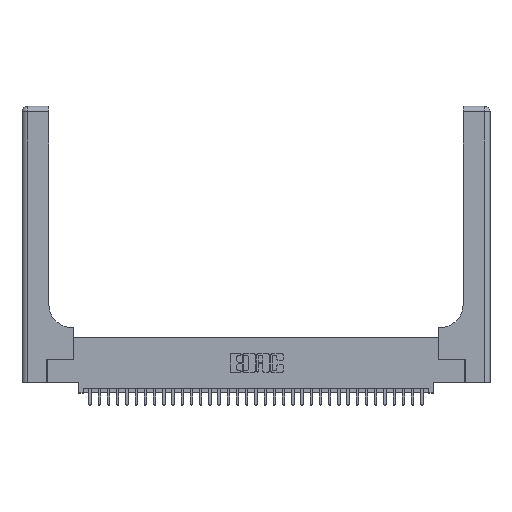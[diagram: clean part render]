
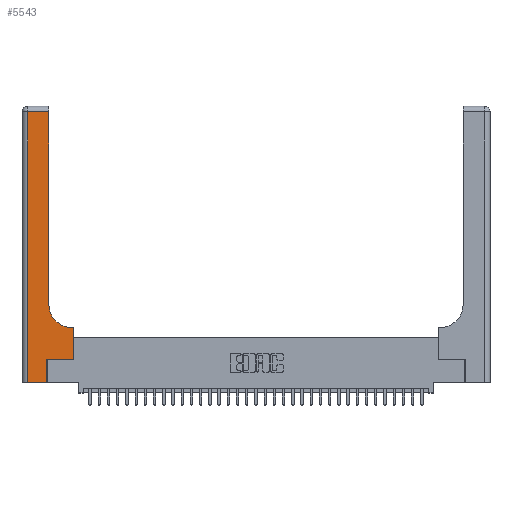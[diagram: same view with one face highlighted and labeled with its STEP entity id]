
A CAD part, top view. The second image highlights one B-rep face of the part: STEP entity #5543.
In plain terms, the highlighted planar face has unit normal (0, 0, 1).
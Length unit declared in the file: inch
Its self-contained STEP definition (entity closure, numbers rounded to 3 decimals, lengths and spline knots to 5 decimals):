
#311 = VECTOR ( 'NONE', #27651, 39.37008 ) ;
#631 = ORIENTED_EDGE ( 'NONE', *, *, #18837, .T. ) ;
#1269 = ORIENTED_EDGE ( 'NONE', *, *, #34056, .T. ) ;
#2179 = ORIENTED_EDGE ( 'NONE', *, *, #4303, .T. ) ;
#2288 = DIRECTION ( 'NONE',  ( 0., -1., 0. ) ) ;
#2708 = EDGE_CURVE ( 'NONE', #18222, #19140, #27101, .T. ) ;
#3225 = VERTEX_POINT ( 'NONE', #10753 ) ;
#3307 = VECTOR ( 'NONE', #16901, 39.37008 ) ;
#3483 = EDGE_LOOP ( 'NONE', ( #31436, #631, #7816, #16513, #2179, #1269, #25852, #31428, #10002 ) ) ;
#3797 = VECTOR ( 'NONE', #31419, 39.37008 ) ;
#4303 = EDGE_CURVE ( 'NONE', #20511, #27950, #19788, .T. ) ;
#4443 = DIRECTION ( 'NONE',  ( -1., 0., 0. ) ) ;
#4477 = LINE ( 'NONE', #28960, #18033 ) ;
#4658 = CARTESIAN_POINT ( 'NONE',  ( 0.2915, 0.85, 0.37 ) ) ;
#4847 = CARTESIAN_POINT ( 'NONE',  ( 0.5585, 0.25, 0.37 ) ) ;
#4899 = FACE_OUTER_BOUND ( 'NONE', #3483, .T. ) ;
#5373 = EDGE_CURVE ( 'NONE', #19140, #12829, #15077, .T. ) ;
#5478 = VECTOR ( 'NONE', #10313, 39.37008 ) ;
#5543 = ADVANCED_FACE ( 'NONE', ( #4899 ), #7149, .F. ) ;
#6125 = CARTESIAN_POINT ( 'NONE',  ( 0.2915, 3., 0.37 ) ) ;
#6303 = CIRCLE ( 'NONE', #25677, 0.25 ) ;
#6802 = DIRECTION ( 'NONE',  ( 0., 0., -1. ) ) ;
#7149 = PLANE ( 'NONE',  #17591 ) ;
#7816 = ORIENTED_EDGE ( 'NONE', *, *, #22633, .T. ) ;
#7909 = VECTOR ( 'NONE', #4443, 39.37008 ) ;
#8424 = LINE ( 'NONE', #16983, #311 ) ;
#9308 = CARTESIAN_POINT ( 'NONE',  ( 0.269, 0.25, 0.37 ) ) ;
#10002 = ORIENTED_EDGE ( 'NONE', *, *, #13266, .T. ) ;
#10313 = DIRECTION ( 'NONE',  ( 0., 1., 0. ) ) ;
#10753 = CARTESIAN_POINT ( 'NONE',  ( 0.2915, 2.94, 0.37 ) ) ;
#12346 = CARTESIAN_POINT ( 'NONE',  ( 0.2915, 0.6, 0.37 ) ) ;
#12829 = VERTEX_POINT ( 'NONE', #26556 ) ;
#13266 = EDGE_CURVE ( 'NONE', #12829, #19223, #6303, .T. ) ;
#13506 = LINE ( 'NONE', #24173, #30046 ) ;
#15077 = LINE ( 'NONE', #12346, #7909 ) ;
#16513 = ORIENTED_EDGE ( 'NONE', *, *, #24229, .T. ) ;
#16901 = DIRECTION ( 'NONE',  ( 0., 1., 0. ) ) ;
#16983 = CARTESIAN_POINT ( 'NONE',  ( 0.269, 0.25, 0.37 ) ) ;
#17591 = AXIS2_PLACEMENT_3D ( 'NONE', #30377, #24160, #24280 ) ;
#18033 = VECTOR ( 'NONE', #20505, 39.37008 ) ;
#18130 = VECTOR ( 'NONE', #29184, 39.37008 ) ;
#18222 = VERTEX_POINT ( 'NONE', #23269 ) ;
#18837 = EDGE_CURVE ( 'NONE', #3225, #25719, #23766, .T. ) ;
#19140 = VERTEX_POINT ( 'NONE', #20725 ) ;
#19223 = VERTEX_POINT ( 'NONE', #4658 ) ;
#19788 = LINE ( 'NONE', #28834, #18130 ) ;
#20505 = DIRECTION ( 'NONE',  ( 1., 0., 0. ) ) ;
#20511 = VERTEX_POINT ( 'NONE', #31640 ) ;
#20725 = CARTESIAN_POINT ( 'NONE',  ( 0.5585, 0.6, 0.37 ) ) ;
#21324 = CARTESIAN_POINT ( 'NONE',  ( 0.06, 2.94, 0.37 ) ) ;
#22633 = EDGE_CURVE ( 'NONE', #25719, #29796, #13506, .T. ) ;
#22905 = DIRECTION ( 'NONE',  ( 1., 0., 0. ) ) ;
#22948 = EDGE_CURVE ( 'NONE', #19223, #3225, #32971, .T. ) ;
#23269 = CARTESIAN_POINT ( 'NONE',  ( 0.5585, 0.25, 0.37 ) ) ;
#23766 = LINE ( 'NONE', #31289, #3797 ) ;
#24160 = DIRECTION ( 'NONE',  ( 0., 0., -1. ) ) ;
#24173 = CARTESIAN_POINT ( 'NONE',  ( 0.06, 3., 0.37 ) ) ;
#24229 = EDGE_CURVE ( 'NONE', #29796, #20511, #4477, .T. ) ;
#24280 = DIRECTION ( 'NONE',  ( -1., 0., 0. ) ) ;
#25677 = AXIS2_PLACEMENT_3D ( 'NONE', #33554, #6802, #22905 ) ;
#25719 = VERTEX_POINT ( 'NONE', #21324 ) ;
#25852 = ORIENTED_EDGE ( 'NONE', *, *, #2708, .T. ) ;
#26556 = CARTESIAN_POINT ( 'NONE',  ( 0.5415, 0.6, 0.37 ) ) ;
#27101 = LINE ( 'NONE', #4847, #5478 ) ;
#27178 = CARTESIAN_POINT ( 'NONE',  ( 0.06, 0., 0.37 ) ) ;
#27651 = DIRECTION ( 'NONE',  ( 1., 0., 0. ) ) ;
#27950 = VERTEX_POINT ( 'NONE', #9308 ) ;
#28834 = CARTESIAN_POINT ( 'NONE',  ( 0.269, 0., 0.37 ) ) ;
#28960 = CARTESIAN_POINT ( 'NONE',  ( 0., 0., 0.37 ) ) ;
#29184 = DIRECTION ( 'NONE',  ( 0., 1., 0. ) ) ;
#29796 = VERTEX_POINT ( 'NONE', #27178 ) ;
#30046 = VECTOR ( 'NONE', #2288, 39.37008 ) ;
#30377 = CARTESIAN_POINT ( 'NONE',  ( 0., 3., 0.37 ) ) ;
#31289 = CARTESIAN_POINT ( 'NONE',  ( 0., 2.94, 0.37 ) ) ;
#31419 = DIRECTION ( 'NONE',  ( -1., 0., 0. ) ) ;
#31428 = ORIENTED_EDGE ( 'NONE', *, *, #5373, .T. ) ;
#31436 = ORIENTED_EDGE ( 'NONE', *, *, #22948, .T. ) ;
#31640 = CARTESIAN_POINT ( 'NONE',  ( 0.269, 0., 0.37 ) ) ;
#32971 = LINE ( 'NONE', #6125, #3307 ) ;
#33554 = CARTESIAN_POINT ( 'NONE',  ( 0.5415, 0.85, 0.37 ) ) ;
#34056 = EDGE_CURVE ( 'NONE', #27950, #18222, #8424, .T. ) ;
